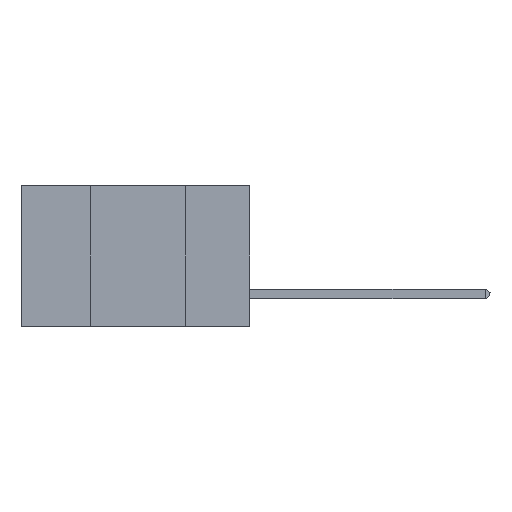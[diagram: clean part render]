
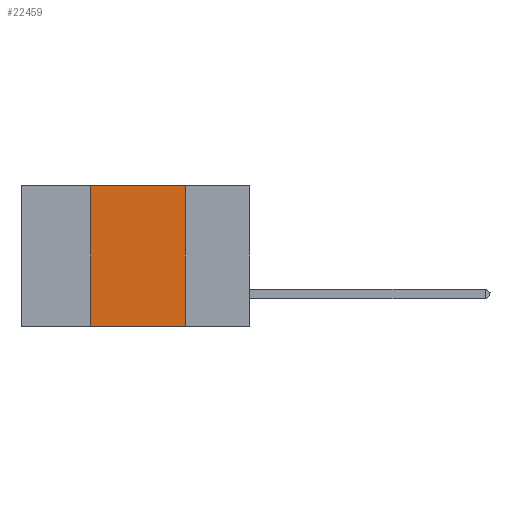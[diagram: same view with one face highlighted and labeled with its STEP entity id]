
A CAD part, left-side view. The second image highlights one B-rep face of the part: STEP entity #22459.
In plain terms, the highlighted planar face has unit normal (-1, 0, 0).
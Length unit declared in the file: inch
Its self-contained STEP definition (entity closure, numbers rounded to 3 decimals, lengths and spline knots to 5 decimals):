
#1582 = ORIENTED_EDGE ( 'NONE', *, *, #27921, .T. ) ;
#4799 = VECTOR ( 'NONE', #26024, 39.37008 ) ;
#5769 = DIRECTION ( 'NONE',  ( 0., 0., -1. ) ) ;
#6971 = DIRECTION ( 'NONE',  ( 0., -1., 0. ) ) ;
#7006 = ORIENTED_EDGE ( 'NONE', *, *, #21242, .F. ) ;
#8866 = AXIS2_PLACEMENT_3D ( 'NONE', #14919, #17946, #35907 ) ;
#10896 = CARTESIAN_POINT ( 'NONE',  ( 0., 0.17, 0. ) ) ;
#12378 = LINE ( 'NONE', #13296, #4799 ) ;
#12562 = CARTESIAN_POINT ( 'NONE',  ( 0., 0.42, -0.37 ) ) ;
#13296 = CARTESIAN_POINT ( 'NONE',  ( 0., 0.42, 0. ) ) ;
#14223 = CARTESIAN_POINT ( 'NONE',  ( 0., 0.42, 0. ) ) ;
#14430 = DIRECTION ( 'NONE',  ( 0., -1., 0. ) ) ;
#14689 = CARTESIAN_POINT ( 'NONE',  ( 0., 0.17, 0. ) ) ;
#14919 = CARTESIAN_POINT ( 'NONE',  ( 0., 0.6, 0. ) ) ;
#17946 = DIRECTION ( 'NONE',  ( 1., 0., 0. ) ) ;
#19765 = EDGE_CURVE ( 'NONE', #21096, #37279, #21154, .T. ) ;
#21096 = VERTEX_POINT ( 'NONE', #14223 ) ;
#21154 = LINE ( 'NONE', #30856, #28196 ) ;
#21242 = EDGE_CURVE ( 'NONE', #33731, #21096, #12378, .T. ) ;
#22459 = ADVANCED_FACE ( 'NONE', ( #37326 ), #27215, .F. ) ;
#26024 = DIRECTION ( 'NONE',  ( 0., 0., 1. ) ) ;
#26919 = VECTOR ( 'NONE', #14430, 39.37008 ) ;
#27215 = PLANE ( 'NONE',  #8866 ) ;
#27270 = EDGE_CURVE ( 'NONE', #37279, #29883, #30716, .T. ) ;
#27473 = ORIENTED_EDGE ( 'NONE', *, *, #27270, .F. ) ;
#27921 = EDGE_CURVE ( 'NONE', #33731, #29883, #39173, .T. ) ;
#28196 = VECTOR ( 'NONE', #6971, 39.37008 ) ;
#29883 = VERTEX_POINT ( 'NONE', #37281 ) ;
#30716 = LINE ( 'NONE', #14689, #31660 ) ;
#30856 = CARTESIAN_POINT ( 'NONE',  ( 0., 0.6, 0. ) ) ;
#31660 = VECTOR ( 'NONE', #5769, 39.37008 ) ;
#32561 = CARTESIAN_POINT ( 'NONE',  ( 0., 0.6, -0.37 ) ) ;
#33731 = VERTEX_POINT ( 'NONE', #12562 ) ;
#35505 = EDGE_LOOP ( 'NONE', ( #27473, #36066, #7006, #1582 ) ) ;
#35907 = DIRECTION ( 'NONE',  ( 0., 0., -1. ) ) ;
#36066 = ORIENTED_EDGE ( 'NONE', *, *, #19765, .F. ) ;
#37279 = VERTEX_POINT ( 'NONE', #10896 ) ;
#37281 = CARTESIAN_POINT ( 'NONE',  ( 0., 0.17, -0.37 ) ) ;
#37326 = FACE_OUTER_BOUND ( 'NONE', #35505, .T. ) ;
#39173 = LINE ( 'NONE', #32561, #26919 ) ;
